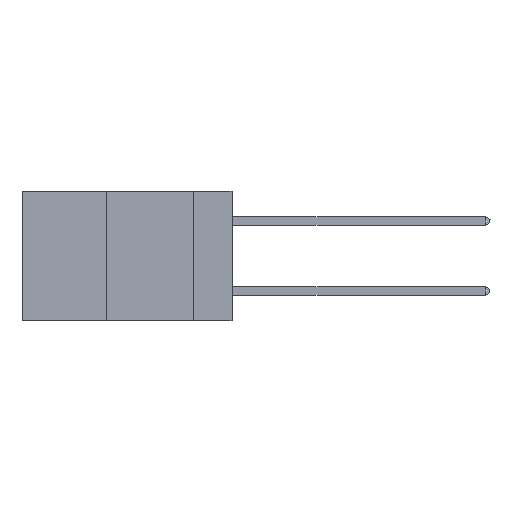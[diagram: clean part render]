
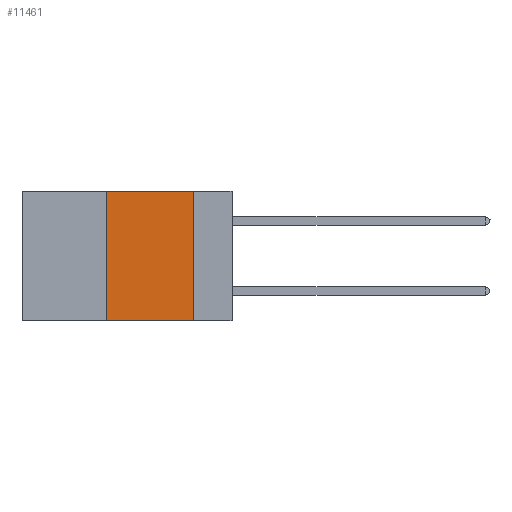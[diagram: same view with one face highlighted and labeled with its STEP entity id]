
A CAD part, left-side view. The second image highlights one B-rep face of the part: STEP entity #11461.
In plain terms, the highlighted planar face has unit normal (-1, 0, 0).
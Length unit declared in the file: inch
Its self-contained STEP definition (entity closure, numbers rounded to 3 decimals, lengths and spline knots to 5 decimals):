
#306 = LINE ( 'NONE', #4268, #14773 ) ;
#478 = CARTESIAN_POINT ( 'NONE',  ( 0., 0.36, 0. ) ) ;
#1135 = CARTESIAN_POINT ( 'NONE',  ( 0., 0.11, -0.37 ) ) ;
#1215 = VECTOR ( 'NONE', #6727, 39.37008 ) ;
#1232 = DIRECTION ( 'NONE',  ( 0., 0., -1. ) ) ;
#1473 = EDGE_CURVE ( 'NONE', #5691, #6909, #306, .T. ) ;
#1889 = DIRECTION ( 'NONE',  ( 1., 0., 0. ) ) ;
#2875 = CARTESIAN_POINT ( 'NONE',  ( 0., 0.6, 0. ) ) ;
#3744 = VECTOR ( 'NONE', #1232, 39.37008 ) ;
#3842 = ORIENTED_EDGE ( 'NONE', *, *, #1473, .T. ) ;
#4268 = CARTESIAN_POINT ( 'NONE',  ( 0., 0.6, -0.37 ) ) ;
#4577 = CARTESIAN_POINT ( 'NONE',  ( 0., 0.36, 0. ) ) ;
#4590 = ORIENTED_EDGE ( 'NONE', *, *, #10929, .F. ) ;
#4937 = CARTESIAN_POINT ( 'NONE',  ( 0., 0.36, -0.37 ) ) ;
#5343 = VERTEX_POINT ( 'NONE', #6182 ) ;
#5350 = CARTESIAN_POINT ( 'NONE',  ( 0., 0.11, 0. ) ) ;
#5691 = VERTEX_POINT ( 'NONE', #4937 ) ;
#6182 = CARTESIAN_POINT ( 'NONE',  ( 0., 0.11, 0. ) ) ;
#6727 = DIRECTION ( 'NONE',  ( 0., -1., 0. ) ) ;
#6909 = VERTEX_POINT ( 'NONE', #1135 ) ;
#7054 = DIRECTION ( 'NONE',  ( 0., 0., -1. ) ) ;
#7612 = EDGE_CURVE ( 'NONE', #5691, #15120, #13908, .T. ) ;
#7683 = AXIS2_PLACEMENT_3D ( 'NONE', #13906, #1889, #7054 ) ;
#9858 = VECTOR ( 'NONE', #13726, 39.37008 ) ;
#10125 = EDGE_CURVE ( 'NONE', #5343, #6909, #14626, .T. ) ;
#10929 = EDGE_CURVE ( 'NONE', #15120, #5343, #13399, .T. ) ;
#11461 = ADVANCED_FACE ( 'NONE', ( #15277 ), #13814, .F. ) ;
#11569 = ORIENTED_EDGE ( 'NONE', *, *, #7612, .F. ) ;
#11673 = EDGE_LOOP ( 'NONE', ( #16345, #4590, #11569, #3842 ) ) ;
#13399 = LINE ( 'NONE', #2875, #1215 ) ;
#13560 = DIRECTION ( 'NONE',  ( 0., -1., 0. ) ) ;
#13726 = DIRECTION ( 'NONE',  ( 0., 0., 1. ) ) ;
#13814 = PLANE ( 'NONE',  #7683 ) ;
#13906 = CARTESIAN_POINT ( 'NONE',  ( 0., 0.6, 0. ) ) ;
#13908 = LINE ( 'NONE', #478, #9858 ) ;
#14626 = LINE ( 'NONE', #5350, #3744 ) ;
#14773 = VECTOR ( 'NONE', #13560, 39.37008 ) ;
#15120 = VERTEX_POINT ( 'NONE', #4577 ) ;
#15277 = FACE_OUTER_BOUND ( 'NONE', #11673, .T. ) ;
#16345 = ORIENTED_EDGE ( 'NONE', *, *, #10125, .F. ) ;
